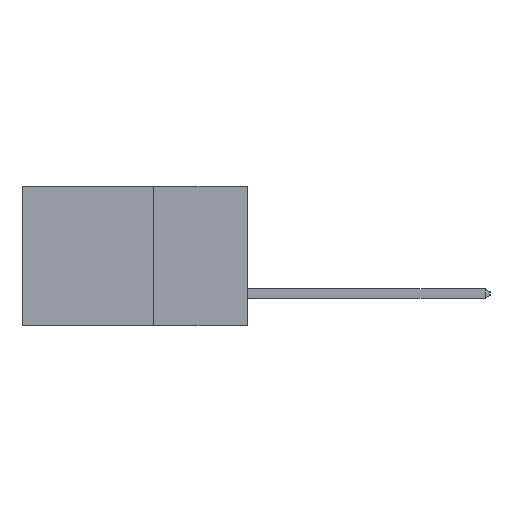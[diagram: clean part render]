
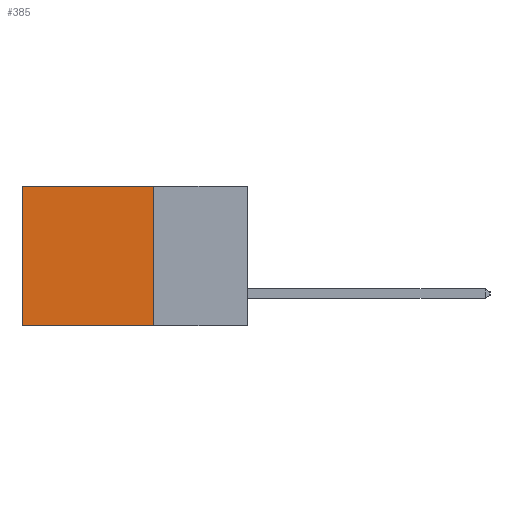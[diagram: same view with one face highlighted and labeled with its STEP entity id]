
A CAD part, left-side view. The second image highlights one B-rep face of the part: STEP entity #385.
In plain terms, the highlighted planar face has unit normal (-1, 0, 0).
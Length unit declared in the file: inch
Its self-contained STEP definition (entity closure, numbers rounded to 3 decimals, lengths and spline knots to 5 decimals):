
#267 = ORIENTED_EDGE ( 'NONE', *, *, #562, .T. ) ;
#385 = ADVANCED_FACE ( 'NONE', ( #10747 ), #7596, .F. ) ;
#562 = EDGE_CURVE ( 'NONE', #10330, #10097, #5012, .T. ) ;
#939 = CARTESIAN_POINT ( 'NONE',  ( 0.298, 0.25, 0. ) ) ;
#1193 = ORIENTED_EDGE ( 'NONE', *, *, #1841, .T. ) ;
#1519 = CARTESIAN_POINT ( 'NONE',  ( 0.298, 0.6, -0.37 ) ) ;
#1841 = EDGE_CURVE ( 'NONE', #10097, #11129, #11973, .T. ) ;
#1869 = VECTOR ( 'NONE', #14392, 39.37008 ) ;
#2027 = EDGE_CURVE ( 'NONE', #8711, #11129, #7005, .T. ) ;
#4454 = EDGE_CURVE ( 'NONE', #10330, #8711, #13186, .T. ) ;
#5012 = LINE ( 'NONE', #939, #1869 ) ;
#5240 = ORIENTED_EDGE ( 'NONE', *, *, #4454, .F. ) ;
#5749 = EDGE_LOOP ( 'NONE', ( #1193, #11220, #5240, #267 ) ) ;
#6289 = DIRECTION ( 'NONE',  ( 0., 0., -1. ) ) ;
#7005 = LINE ( 'NONE', #11501, #12839 ) ;
#7596 = PLANE ( 'NONE',  #14634 ) ;
#8711 = VERTEX_POINT ( 'NONE', #11322 ) ;
#8725 = DIRECTION ( 'NONE',  ( 0., 1., 0. ) ) ;
#8832 = CARTESIAN_POINT ( 'NONE',  ( 0.298, 0.25, 0. ) ) ;
#8853 = VECTOR ( 'NONE', #8953, 39.37008 ) ;
#8953 = DIRECTION ( 'NONE',  ( 0., 0., -1. ) ) ;
#8967 = DIRECTION ( 'NONE',  ( 1., 0., 0. ) ) ;
#8999 = DIRECTION ( 'NONE',  ( 0., 0., -1. ) ) ;
#9383 = CARTESIAN_POINT ( 'NONE',  ( 0.298, 0.6, 0. ) ) ;
#9769 = VECTOR ( 'NONE', #6289, 39.37008 ) ;
#10097 = VERTEX_POINT ( 'NONE', #13826 ) ;
#10330 = VERTEX_POINT ( 'NONE', #12795 ) ;
#10747 = FACE_OUTER_BOUND ( 'NONE', #5749, .T. ) ;
#11129 = VERTEX_POINT ( 'NONE', #1519 ) ;
#11220 = ORIENTED_EDGE ( 'NONE', *, *, #2027, .F. ) ;
#11322 = CARTESIAN_POINT ( 'NONE',  ( 0.298, 0.25, -0.37 ) ) ;
#11501 = CARTESIAN_POINT ( 'NONE',  ( 0.298, 0.25, -0.37 ) ) ;
#11973 = LINE ( 'NONE', #9383, #8853 ) ;
#12795 = CARTESIAN_POINT ( 'NONE',  ( 0.298, 0.25, 0. ) ) ;
#12839 = VECTOR ( 'NONE', #8725, 39.37008 ) ;
#13186 = LINE ( 'NONE', #14321, #9769 ) ;
#13826 = CARTESIAN_POINT ( 'NONE',  ( 0.298, 0.6, 0. ) ) ;
#14321 = CARTESIAN_POINT ( 'NONE',  ( 0.298, 0.25, 0. ) ) ;
#14392 = DIRECTION ( 'NONE',  ( 0., 1., 0. ) ) ;
#14634 = AXIS2_PLACEMENT_3D ( 'NONE', #8832, #8967, #8999 ) ;
